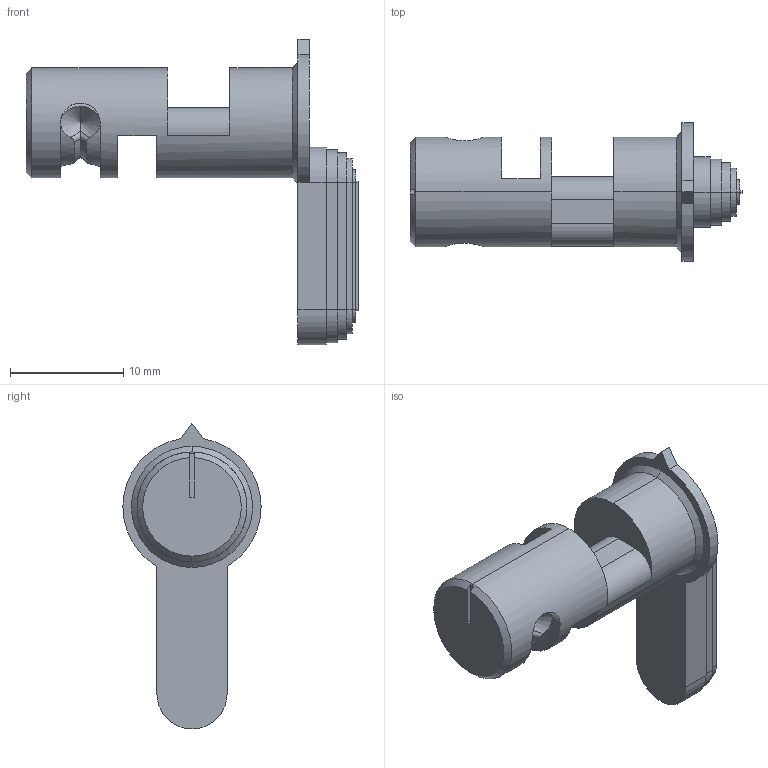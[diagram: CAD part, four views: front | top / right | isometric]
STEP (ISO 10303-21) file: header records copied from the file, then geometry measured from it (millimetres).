
FILE_DESCRIPTION (( 'STEP AP203' ), '1' );
FILE_NAME ('selector.STEP', '2021-12-29T04:19:11', ( '' ), ( '' ), 'SwSTEP 2.0', 'SolidWorks 2015', '' );
FILE_SCHEMA (( 'CONFIG_CONTROL_DESIGN' ));
Length unit declared in the file: millimetre
Products named in the file (1): selector
Bounding box: 29.3 x 12.2 x 27 mm (x, y, z)
Volume: 1860.7 mm3; surface area: 1471.6 mm2
Topology: 1 solids, 1 shells, 93 faces, 240 edges, 149 vertices
Faces by surface type: plane 37, cylinder 34, cone 14, bspline 8
Entity records: 3219 total; most frequent: CARTESIAN_POINT 969, ORIENTED_EDGE 468, DIRECTION 436, EDGE_CURVE 234, AXIS2_PLACEMENT_3D 164, VERTEX_POINT 149, LINE 108, VECTOR 108
